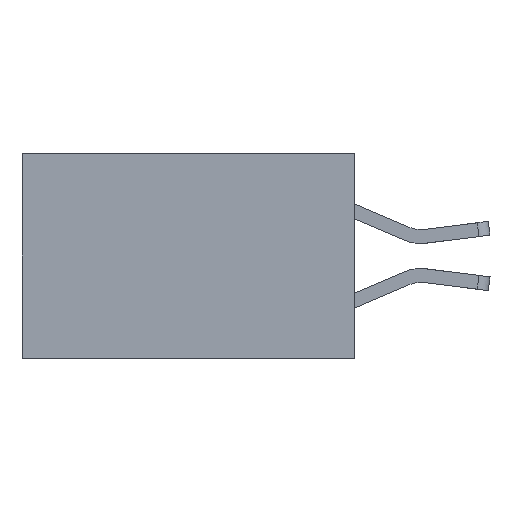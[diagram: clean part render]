
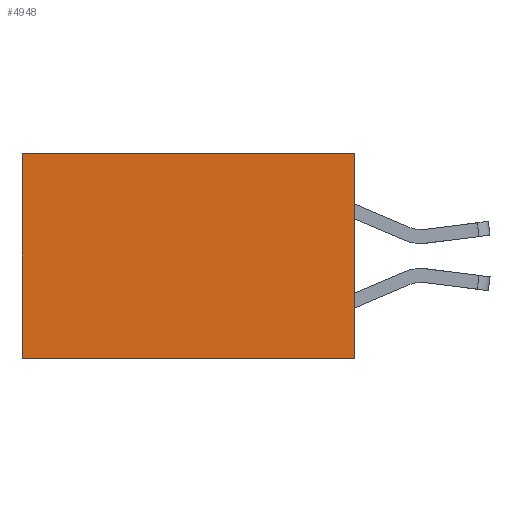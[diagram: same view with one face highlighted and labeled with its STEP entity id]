
A CAD part, left-side view. The second image highlights one B-rep face of the part: STEP entity #4948.
In plain terms, the highlighted planar face has unit normal (-1, 0, 0).
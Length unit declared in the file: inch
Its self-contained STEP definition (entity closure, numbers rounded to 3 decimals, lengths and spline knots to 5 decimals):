
#220 = CARTESIAN_POINT ( 'NONE',  ( 0.298, 0., 0. ) ) ;
#656 = VECTOR ( 'NONE', #6428, 39.37008 ) ;
#902 = LINE ( 'NONE', #5611, #7737 ) ;
#930 = PLANE ( 'NONE',  #4058 ) ;
#1239 = EDGE_CURVE ( 'NONE', #10885, #3434, #5857, .T. ) ;
#1268 = DIRECTION ( 'NONE',  ( 0., 0., -1. ) ) ;
#1286 = DIRECTION ( 'NONE',  ( 0., 0., -1. ) ) ;
#1490 = CARTESIAN_POINT ( 'NONE',  ( 0.298, 0.6, -0.37 ) ) ;
#2444 = ORIENTED_EDGE ( 'NONE', *, *, #7389, .F. ) ;
#2992 = VERTEX_POINT ( 'NONE', #7009 ) ;
#3154 = EDGE_LOOP ( 'NONE', ( #8554, #6565, #2444, #3198 ) ) ;
#3198 = ORIENTED_EDGE ( 'NONE', *, *, #5881, .T. ) ;
#3434 = VERTEX_POINT ( 'NONE', #1490 ) ;
#3443 = DIRECTION ( 'NONE',  ( 0., 0., -1. ) ) ;
#3528 = VECTOR ( 'NONE', #1268, 39.37008 ) ;
#3934 = LINE ( 'NONE', #7384, #10626 ) ;
#4058 = AXIS2_PLACEMENT_3D ( 'NONE', #6890, #9500, #3443 ) ;
#4267 = VERTEX_POINT ( 'NONE', #8137 ) ;
#4875 = CARTESIAN_POINT ( 'NONE',  ( 0.298, 0.6, 0. ) ) ;
#4878 = DIRECTION ( 'NONE',  ( 0., 1., 0. ) ) ;
#4948 = ADVANCED_FACE ( 'NONE', ( #8881 ), #930, .F. ) ;
#5611 = CARTESIAN_POINT ( 'NONE',  ( 0.298, 0., 0. ) ) ;
#5628 = CARTESIAN_POINT ( 'NONE',  ( 0.298, 0.6, 0. ) ) ;
#5857 = LINE ( 'NONE', #5628, #3528 ) ;
#5881 = EDGE_CURVE ( 'NONE', #4267, #10885, #7636, .T. ) ;
#6428 = DIRECTION ( 'NONE',  ( 0., 1., 0. ) ) ;
#6565 = ORIENTED_EDGE ( 'NONE', *, *, #6672, .F. ) ;
#6672 = EDGE_CURVE ( 'NONE', #2992, #3434, #3934, .T. ) ;
#6890 = CARTESIAN_POINT ( 'NONE',  ( 0.298, 0., 0. ) ) ;
#7009 = CARTESIAN_POINT ( 'NONE',  ( 0.298, 0., -0.37 ) ) ;
#7384 = CARTESIAN_POINT ( 'NONE',  ( 0.298, 0., -0.37 ) ) ;
#7389 = EDGE_CURVE ( 'NONE', #4267, #2992, #902, .T. ) ;
#7636 = LINE ( 'NONE', #220, #656 ) ;
#7737 = VECTOR ( 'NONE', #1286, 39.37008 ) ;
#8137 = CARTESIAN_POINT ( 'NONE',  ( 0.298, 0., 0. ) ) ;
#8554 = ORIENTED_EDGE ( 'NONE', *, *, #1239, .T. ) ;
#8881 = FACE_OUTER_BOUND ( 'NONE', #3154, .T. ) ;
#9500 = DIRECTION ( 'NONE',  ( 1., 0., 0. ) ) ;
#10626 = VECTOR ( 'NONE', #4878, 39.37008 ) ;
#10885 = VERTEX_POINT ( 'NONE', #4875 ) ;
